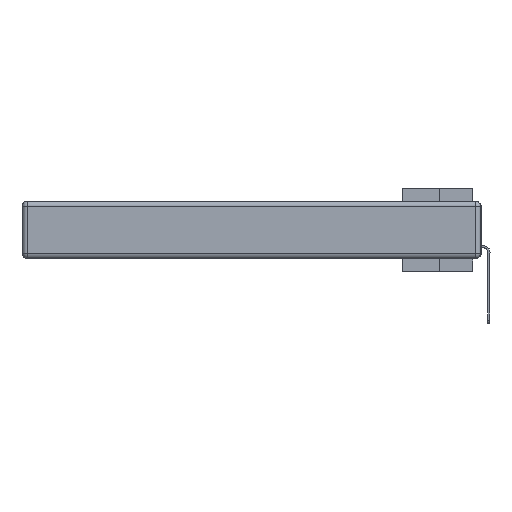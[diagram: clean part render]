
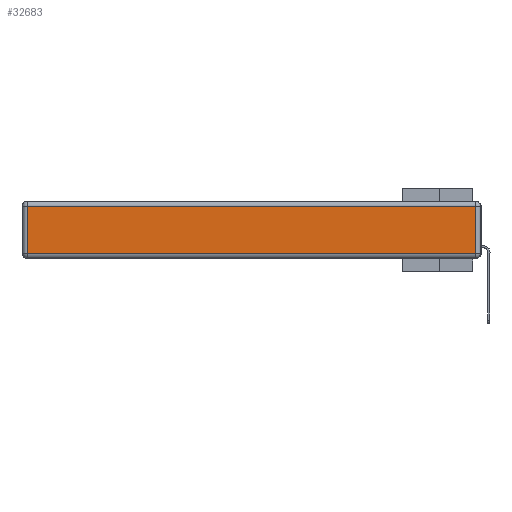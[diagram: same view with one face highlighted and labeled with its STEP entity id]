
A CAD part, left-side view. The second image highlights one B-rep face of the part: STEP entity #32683.
In plain terms, the highlighted planar face has unit normal (-1, 0, 0).
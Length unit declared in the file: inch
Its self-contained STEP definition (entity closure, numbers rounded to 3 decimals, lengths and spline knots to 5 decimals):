
#66 = VECTOR ( 'NONE', #21951, 39.37008 ) ;
#626 = AXIS2_PLACEMENT_3D ( 'NONE', #19465, #16812, #5624 ) ;
#2637 = VECTOR ( 'NONE', #30017, 39.37008 ) ;
#4990 = VERTEX_POINT ( 'NONE', #28413 ) ;
#5269 = EDGE_CURVE ( 'NONE', #7930, #22256, #12670, .T. ) ;
#5624 = DIRECTION ( 'NONE',  ( 0., 0., 1. ) ) ;
#5774 = EDGE_CURVE ( 'NONE', #27009, #7930, #22189, .T. ) ;
#5915 = LINE ( 'NONE', #18518, #6372 ) ;
#6372 = VECTOR ( 'NONE', #13064, 39.37008 ) ;
#7729 = CARTESIAN_POINT ( 'NONE',  ( 0., 2.72, -0.03 ) ) ;
#7930 = VERTEX_POINT ( 'NONE', #16762 ) ;
#7977 = CARTESIAN_POINT ( 'NONE',  ( 0., 0., -0.313 ) ) ;
#9811 = ORIENTED_EDGE ( 'NONE', *, *, #5774, .T. ) ;
#11368 = CARTESIAN_POINT ( 'NONE',  ( 0., 0.03, -0.313 ) ) ;
#12670 = LINE ( 'NONE', #7977, #66 ) ;
#13064 = DIRECTION ( 'NONE',  ( 0., 0., 1. ) ) ;
#13176 = CARTESIAN_POINT ( 'NONE',  ( 0., 2.72, -0.343 ) ) ;
#13185 = EDGE_LOOP ( 'NONE', ( #26398, #35865, #34319, #9811 ) ) ;
#13947 = FACE_OUTER_BOUND ( 'NONE', #13185, .T. ) ;
#16762 = CARTESIAN_POINT ( 'NONE',  ( 0., 2.72, -0.313 ) ) ;
#16812 = DIRECTION ( 'NONE',  ( -1., 0., 0. ) ) ;
#18209 = VECTOR ( 'NONE', #33026, 39.37008 ) ;
#18518 = CARTESIAN_POINT ( 'NONE',  ( 0., 0.03, -0.343 ) ) ;
#19465 = CARTESIAN_POINT ( 'NONE',  ( 0., 0., -0.343 ) ) ;
#21951 = DIRECTION ( 'NONE',  ( 0., -1., 0. ) ) ;
#22189 = LINE ( 'NONE', #13176, #2637 ) ;
#22256 = VERTEX_POINT ( 'NONE', #11368 ) ;
#22404 = PLANE ( 'NONE',  #626 ) ;
#26398 = ORIENTED_EDGE ( 'NONE', *, *, #5269, .T. ) ;
#27009 = VERTEX_POINT ( 'NONE', #7729 ) ;
#28413 = CARTESIAN_POINT ( 'NONE',  ( 0., 0.03, -0.03 ) ) ;
#28893 = EDGE_CURVE ( 'NONE', #22256, #4990, #5915, .T. ) ;
#30017 = DIRECTION ( 'NONE',  ( 0., 0., -1. ) ) ;
#31652 = LINE ( 'NONE', #32558, #18209 ) ;
#32558 = CARTESIAN_POINT ( 'NONE',  ( 0., 2.75, -0.03 ) ) ;
#32683 = ADVANCED_FACE ( 'NONE', ( #13947 ), #22404, .T. ) ;
#33026 = DIRECTION ( 'NONE',  ( 0., 1., 0. ) ) ;
#33257 = EDGE_CURVE ( 'NONE', #4990, #27009, #31652, .T. ) ;
#34319 = ORIENTED_EDGE ( 'NONE', *, *, #33257, .T. ) ;
#35865 = ORIENTED_EDGE ( 'NONE', *, *, #28893, .T. ) ;
